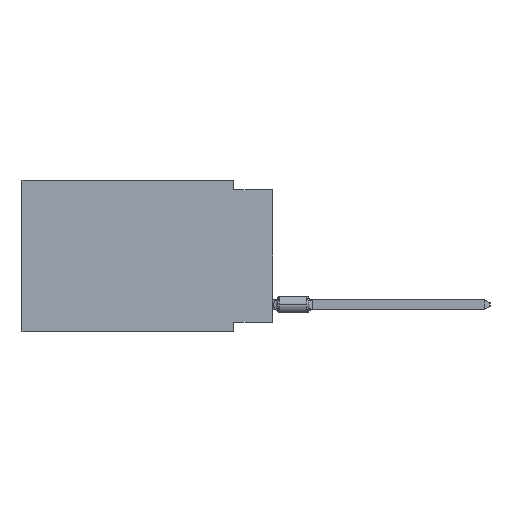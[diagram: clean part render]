
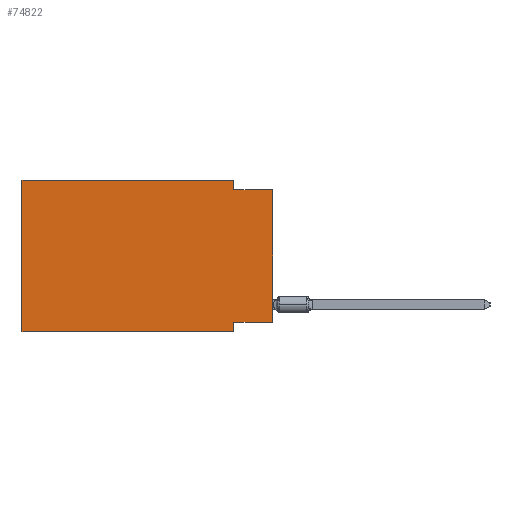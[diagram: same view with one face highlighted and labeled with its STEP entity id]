
A CAD part, left-side view. The second image highlights one B-rep face of the part: STEP entity #74822.
In plain terms, the highlighted planar face has unit normal (-1, 0, 0).
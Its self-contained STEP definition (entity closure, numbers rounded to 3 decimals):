
#308 = ORIENTED_EDGE ( 'NONE', *, *, #2136, .F. ) ;
#959 = ORIENTED_EDGE ( 'NONE', *, *, #53228, .T. ) ;
#1258 = VERTEX_POINT ( 'NONE', #86340 ) ;
#2136 = EDGE_CURVE ( 'NONE', #5595, #30882, #87020, .T. ) ;
#5308 = VECTOR ( 'NONE', #12451, 1000. ) ;
#5595 = VERTEX_POINT ( 'NONE', #83788 ) ;
#12451 = DIRECTION ( 'NONE',  ( 0., -1., 0. ) ) ;
#13966 = LINE ( 'NONE', #68317, #16654 ) ;
#16654 = VECTOR ( 'NONE', #47805, 1000. ) ;
#18367 = DIRECTION ( 'NONE',  ( 0., 0., -1. ) ) ;
#20317 = EDGE_CURVE ( 'NONE', #86928, #23194, #45975, .T. ) ;
#23194 = VERTEX_POINT ( 'NONE', #34850 ) ;
#25979 = VERTEX_POINT ( 'NONE', #76189 ) ;
#26521 = CARTESIAN_POINT ( 'NONE',  ( 0., 2.54, 0. ) ) ;
#26867 = CARTESIAN_POINT ( 'NONE',  ( 0., 2.54, -9.271 ) ) ;
#27210 = CARTESIAN_POINT ( 'NONE',  ( 0., 0., -9.271 ) ) ;
#27682 = CARTESIAN_POINT ( 'NONE',  ( 0., 16.383, 0. ) ) ;
#28944 = VERTEX_POINT ( 'NONE', #85224 ) ;
#30882 = VERTEX_POINT ( 'NONE', #48606 ) ;
#31836 = LINE ( 'NONE', #57706, #49083 ) ;
#31906 = DIRECTION ( 'NONE',  ( 1., 0., 0. ) ) ;
#33350 = EDGE_CURVE ( 'NONE', #49078, #28944, #47881, .T. ) ;
#34850 = CARTESIAN_POINT ( 'NONE',  ( 0., 2.54, -9.906 ) ) ;
#37492 = EDGE_CURVE ( 'NONE', #25979, #86928, #82022, .T. ) ;
#38648 = ORIENTED_EDGE ( 'NONE', *, *, #20317, .F. ) ;
#39298 = ORIENTED_EDGE ( 'NONE', *, *, #52969, .F. ) ;
#39664 = VECTOR ( 'NONE', #75069, 1000. ) ;
#40240 = EDGE_CURVE ( 'NONE', #5595, #23194, #55633, .T. ) ;
#40894 = LINE ( 'NONE', #73471, #5308 ) ;
#43331 = VECTOR ( 'NONE', #60266, 1000. ) ;
#43999 = DIRECTION ( 'NONE',  ( 0., 1., 0. ) ) ;
#45975 = LINE ( 'NONE', #79405, #59231 ) ;
#47805 = DIRECTION ( 'NONE',  ( 0., 0., 1. ) ) ;
#47881 = LINE ( 'NONE', #26521, #39664 ) ;
#48606 = CARTESIAN_POINT ( 'NONE',  ( 0., 16.383, 0. ) ) ;
#48955 = CARTESIAN_POINT ( 'NONE',  ( 0., 16.383, -9.906 ) ) ;
#49078 = VERTEX_POINT ( 'NONE', #85965 ) ;
#49083 = VECTOR ( 'NONE', #62427, 1000. ) ;
#52969 = EDGE_CURVE ( 'NONE', #28944, #1258, #40894, .T. ) ;
#53228 = EDGE_CURVE ( 'NONE', #25979, #1258, #13966, .T. ) ;
#54406 = ORIENTED_EDGE ( 'NONE', *, *, #40240, .T. ) ;
#55633 = LINE ( 'NONE', #48955, #84358 ) ;
#56373 = ORIENTED_EDGE ( 'NONE', *, *, #72892, .F. ) ;
#57706 = CARTESIAN_POINT ( 'NONE',  ( 0., 16.383, 0. ) ) ;
#59231 = VECTOR ( 'NONE', #18367, 1000. ) ;
#60266 = DIRECTION ( 'NONE',  ( 0., 0., 1. ) ) ;
#62427 = DIRECTION ( 'NONE',  ( 0., -1., 0. ) ) ;
#65795 = FACE_OUTER_BOUND ( 'NONE', #70239, .T. ) ;
#68177 = DIRECTION ( 'NONE',  ( 0., -1., 0. ) ) ;
#68317 = CARTESIAN_POINT ( 'NONE',  ( 0., 0., 0. ) ) ;
#68955 = AXIS2_PLACEMENT_3D ( 'NONE', #71597, #31906, #86745 ) ;
#70239 = EDGE_LOOP ( 'NONE', ( #959, #39298, #77541, #56373, #308, #54406, #38648, #87548 ) ) ;
#71597 = CARTESIAN_POINT ( 'NONE',  ( 0., 16.383, 0. ) ) ;
#72892 = EDGE_CURVE ( 'NONE', #30882, #49078, #31836, .T. ) ;
#73344 = PLANE ( 'NONE',  #68955 ) ;
#73471 = CARTESIAN_POINT ( 'NONE',  ( 0., 0., -0.635 ) ) ;
#74822 = ADVANCED_FACE ( 'NONE', ( #65795 ), #73344, .F. ) ;
#75069 = DIRECTION ( 'NONE',  ( 0., 0., -1. ) ) ;
#76189 = CARTESIAN_POINT ( 'NONE',  ( 0., 0., -9.271 ) ) ;
#77541 = ORIENTED_EDGE ( 'NONE', *, *, #33350, .F. ) ;
#79405 = CARTESIAN_POINT ( 'NONE',  ( 0., 2.54, -9.906 ) ) ;
#81283 = VECTOR ( 'NONE', #43999, 1000. ) ;
#82022 = LINE ( 'NONE', #27210, #81283 ) ;
#83788 = CARTESIAN_POINT ( 'NONE',  ( 0., 16.383, -9.906 ) ) ;
#84358 = VECTOR ( 'NONE', #68177, 1000. ) ;
#85224 = CARTESIAN_POINT ( 'NONE',  ( 0., 2.54, -0.635 ) ) ;
#85965 = CARTESIAN_POINT ( 'NONE',  ( 0., 2.54, 0. ) ) ;
#86340 = CARTESIAN_POINT ( 'NONE',  ( 0., 0., -0.635 ) ) ;
#86745 = DIRECTION ( 'NONE',  ( 0., 0., -1. ) ) ;
#86928 = VERTEX_POINT ( 'NONE', #26867 ) ;
#87020 = LINE ( 'NONE', #27682, #43331 ) ;
#87548 = ORIENTED_EDGE ( 'NONE', *, *, #37492, .F. ) ;
